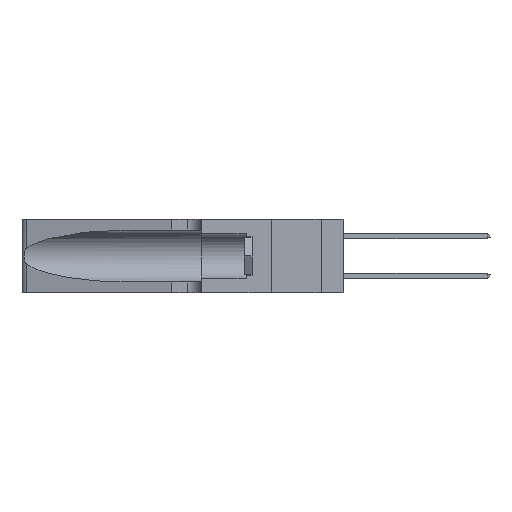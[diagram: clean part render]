
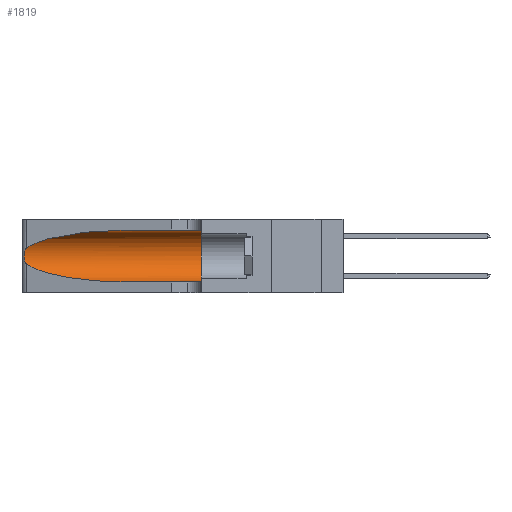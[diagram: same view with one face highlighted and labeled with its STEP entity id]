
A CAD part, left-side view. The second image highlights one B-rep face of the part: STEP entity #1819.
In plain terms, the highlighted cylindrical face has radius 3.308 mm (diameter 6.617 mm), a partial arc.
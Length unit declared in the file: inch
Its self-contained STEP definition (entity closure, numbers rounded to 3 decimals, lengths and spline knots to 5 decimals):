
#43 = VECTOR ( 'NONE', #11450, 39.37008 ) ;
#710 = CARTESIAN_POINT ( 'NONE',  ( 0.1305, 0.72297, 0.31525 ) ) ;
#915 = VERTEX_POINT ( 'NONE', #8245 ) ;
#1819 = ADVANCED_FACE ( 'NONE', ( #16797 ), #36107, .F. ) ;
#2038 =( BOUNDED_CURVE ( )  B_SPLINE_CURVE ( 3, ( #17457, #48317, #25244, #2071 ),
 .UNSPECIFIED., .F., .F. ) 
 B_SPLINE_CURVE_WITH_KNOTS ( ( 4, 4 ),
 ( 3.44316, 4.71239 ),
 .UNSPECIFIED. ) 
 CURVE ( )  GEOMETRIC_REPRESENTATION_ITEM ( )  RATIONAL_B_SPLINE_CURVE ( ( 1., 0.87, 0.87, 1. ) ) 
 REPRESENTATION_ITEM ( '' )  );
#2071 = CARTESIAN_POINT ( 'NONE',  ( 0.1305, 0.72297, 0.05475 ) ) ;
#2334 = CARTESIAN_POINT ( 'NONE',  ( 0.26075, 1.23896, 0.178 ) ) ;
#6177 = VERTEX_POINT ( 'NONE', #39800 ) ;
#6269 = CARTESIAN_POINT ( 'NONE',  ( 0.25856, 1.23593, 0.16098 ) ) ;
#6505 = CIRCLE ( 'NONE', #17753, 0.13025 ) ;
#8245 = CARTESIAN_POINT ( 'NONE',  ( 0.1305, 0.72297, 0.05475 ) ) ;
#10131 = CARTESIAN_POINT ( 'NONE',  ( 0.25639, 1.23186, 0.15144 ) ) ;
#11450 = DIRECTION ( 'NONE',  ( 0., -1., 0. ) ) ;
#14030 = CARTESIAN_POINT ( 'NONE',  ( 0.25487, 1.22718, 0.14631 ) ) ;
#14189 = DIRECTION ( 'NONE',  ( 0., 1., 0. ) ) ;
#16797 = FACE_OUTER_BOUND ( 'NONE', #25163, .T. ) ;
#17457 = CARTESIAN_POINT ( 'NONE',  ( 0.25487, 1.22718, 0.14631 ) ) ;
#17738 = CARTESIAN_POINT ( 'NONE',  ( 0.25639, 1.23184, 0.21858 ) ) ;
#17753 = AXIS2_PLACEMENT_3D ( 'NONE', #37296, #14189, #41163 ) ;
#18562 = EDGE_CURVE ( 'NONE', #6177, #915, #2038, .T. ) ;
#19078 = VERTEX_POINT ( 'NONE', #20618 ) ;
#19226 = EDGE_CURVE ( 'NONE', #40567, #6177, #34247, .T. ) ;
#19956 = CARTESIAN_POINT ( 'NONE',  ( 0.25487, 1.22718, 0.22369 ) ) ;
#20159 = CARTESIAN_POINT ( 'NONE',  ( 0.25487, 1.22718, 0.22369 ) ) ;
#20618 = CARTESIAN_POINT ( 'NONE',  ( 0.1305, 0.35, 0.05475 ) ) ;
#21497 = CARTESIAN_POINT ( 'NONE',  ( 0.1305, 1.61858, 0.185 ) ) ;
#21499 = ORIENTED_EDGE ( 'NONE', *, *, #31960, .T. ) ;
#21611 = CARTESIAN_POINT ( 'NONE',  ( 0.25854, 1.2359, 0.20912 ) ) ;
#21813 = LINE ( 'NONE', #26680, #43 ) ;
#22286 = EDGE_CURVE ( 'NONE', #915, #19078, #21813, .T. ) ;
#24942 = VERTEX_POINT ( 'NONE', #42962 ) ;
#25113 = CARTESIAN_POINT ( 'NONE',  ( 0.1305, 0.35, 0.31525 ) ) ;
#25163 = EDGE_LOOP ( 'NONE', ( #21499, #47491, #27058, #39045, #45550, #34182 ) ) ;
#25244 = CARTESIAN_POINT ( 'NONE',  ( 0.18966, 0.96281, 0.05475 ) ) ;
#25521 = CARTESIAN_POINT ( 'NONE',  ( 0.26075, 1.23896, 0.19203 ) ) ;
#26680 = CARTESIAN_POINT ( 'NONE',  ( 0.1305, 1.61858, 0.05475 ) ) ;
#27058 = ORIENTED_EDGE ( 'NONE', *, *, #18562, .T. ) ;
#29085 = EDGE_CURVE ( 'NONE', #49013, #19078, #6505, .T. ) ;
#29228 = CARTESIAN_POINT ( 'NONE',  ( 0.25555, 1.22994, 0.2215 ) ) ;
#29395 = CARTESIAN_POINT ( 'NONE',  ( 0.26017, 1.23833, 0.17102 ) ) ;
#29978 = AXIS2_PLACEMENT_3D ( 'NONE', #21497, #40761, #48491 ) ;
#31650 = CARTESIAN_POINT ( 'NONE',  ( 0.18966, 0.96281, 0.31525 ) ) ;
#31960 = EDGE_CURVE ( 'NONE', #24942, #40567, #48453, .T. ) ;
#33086 = CARTESIAN_POINT ( 'NONE',  ( 0.25487, 1.22718, 0.22369 ) ) ;
#33256 = CARTESIAN_POINT ( 'NONE',  ( 0.25789, 1.23486, 0.15765 ) ) ;
#33594 = DIRECTION ( 'NONE',  ( 0., -1., 0. ) ) ;
#34182 = ORIENTED_EDGE ( 'NONE', *, *, #38543, .F. ) ;
#34247 = B_SPLINE_CURVE_WITH_KNOTS ( 'NONE', 3,
 ( #33086, #29228, #17738, #44722, #21611, #48590, #25521, #2334, #29395, #6269, #33256, #10131, #37137, #14030 ),
 .UNSPECIFIED., .F., .F.,
 ( 4, 2, 2, 2, 2, 2, 4 ),
 ( 0., 0.00027, 0.00053, 0.00107, 0.0016, 0.00187, 0.00214 ),
 .UNSPECIFIED. ) ;
#36107 = CYLINDRICAL_SURFACE ( 'NONE', #29978, 0.13025 ) ;
#36429 = VECTOR ( 'NONE', #33594, 39.37008 ) ;
#37137 = CARTESIAN_POINT ( 'NONE',  ( 0.25555, 1.22993, 0.14849 ) ) ;
#37296 = CARTESIAN_POINT ( 'NONE',  ( 0.1305, 0.35, 0.185 ) ) ;
#38543 = EDGE_CURVE ( 'NONE', #24942, #49013, #46693, .T. ) ;
#39045 = ORIENTED_EDGE ( 'NONE', *, *, #22286, .T. ) ;
#39800 = CARTESIAN_POINT ( 'NONE',  ( 0.25487, 1.22718, 0.14631 ) ) ;
#40567 = VERTEX_POINT ( 'NONE', #19956 ) ;
#40761 = DIRECTION ( 'NONE',  ( 0., -1., 0. ) ) ;
#41163 = DIRECTION ( 'NONE',  ( 0., 0., 1. ) ) ;
#42962 = CARTESIAN_POINT ( 'NONE',  ( 0.1305, 0.72297, 0.31525 ) ) ;
#43273 = CARTESIAN_POINT ( 'NONE',  ( 0.2373, 1.15595, 0.28018 ) ) ;
#44722 = CARTESIAN_POINT ( 'NONE',  ( 0.25787, 1.23484, 0.2124 ) ) ;
#45051 = CARTESIAN_POINT ( 'NONE',  ( 0.1305, 1.61858, 0.31525 ) ) ;
#45550 = ORIENTED_EDGE ( 'NONE', *, *, #29085, .F. ) ;
#46693 = LINE ( 'NONE', #45051, #36429 ) ;
#47491 = ORIENTED_EDGE ( 'NONE', *, *, #19226, .T. ) ;
#48317 = CARTESIAN_POINT ( 'NONE',  ( 0.2373, 1.15595, 0.08982 ) ) ;
#48453 =( BOUNDED_CURVE ( )  B_SPLINE_CURVE ( 3, ( #710, #31650, #43273, #20159 ),
 .UNSPECIFIED., .F., .T. ) 
 B_SPLINE_CURVE_WITH_KNOTS ( ( 4, 4 ),
 ( 1.5708, 2.84003 ),
 .UNSPECIFIED. ) 
 CURVE ( )  GEOMETRIC_REPRESENTATION_ITEM ( )  RATIONAL_B_SPLINE_CURVE ( ( 1., 0.87, 0.87, 1. ) ) 
 REPRESENTATION_ITEM ( '' )  );
#48491 = DIRECTION ( 'NONE',  ( 0., 0., -1. ) ) ;
#48590 = CARTESIAN_POINT ( 'NONE',  ( 0.26018, 1.23835, 0.19895 ) ) ;
#49013 = VERTEX_POINT ( 'NONE', #25113 ) ;
